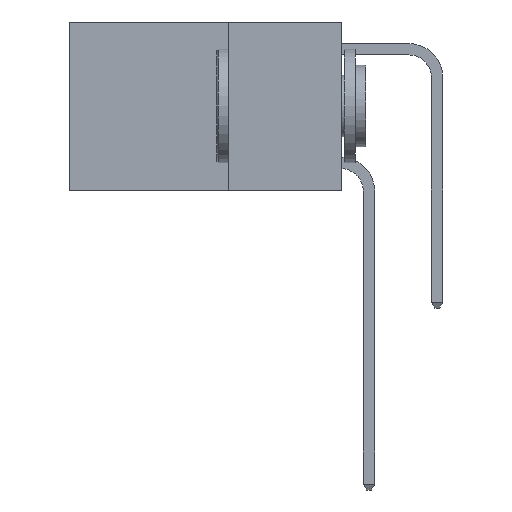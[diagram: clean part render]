
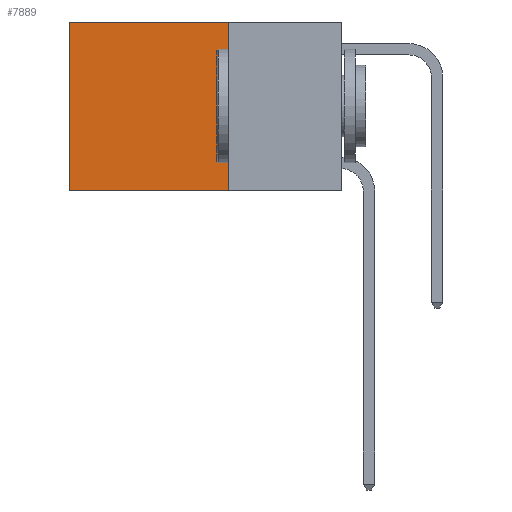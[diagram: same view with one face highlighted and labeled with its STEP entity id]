
A CAD part, left-side view. The second image highlights one B-rep face of the part: STEP entity #7889.
In plain terms, the highlighted planar face has unit normal (-1, 0, 0).
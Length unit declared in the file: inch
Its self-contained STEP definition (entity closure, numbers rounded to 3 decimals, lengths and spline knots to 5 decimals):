
#474 = DIRECTION ( 'NONE',  ( 0., 1., 0. ) ) ;
#716 = AXIS2_PLACEMENT_3D ( 'NONE', #8665, #10063, #4772 ) ;
#807 = PLANE ( 'NONE',  #716 ) ;
#1109 = VERTEX_POINT ( 'NONE', #6477 ) ;
#1209 = EDGE_CURVE ( 'NONE', #4721, #1109, #2411, .T. ) ;
#1441 = ORIENTED_EDGE ( 'NONE', *, *, #4058, .T. ) ;
#1453 = VECTOR ( 'NONE', #474, 39.37008 ) ;
#2411 = LINE ( 'NONE', #10337, #1453 ) ;
#2721 = ORIENTED_EDGE ( 'NONE', *, *, #1209, .F. ) ;
#2748 = EDGE_LOOP ( 'NONE', ( #1441, #2721, #3820, #3314 ) ) ;
#3028 = CARTESIAN_POINT ( 'NONE',  ( 0.2625, 0.25, 0. ) ) ;
#3314 = ORIENTED_EDGE ( 'NONE', *, *, #4713, .T. ) ;
#3820 = ORIENTED_EDGE ( 'NONE', *, *, #5455, .F. ) ;
#3892 = CARTESIAN_POINT ( 'NONE',  ( 0.2625, 0.25, 0. ) ) ;
#4058 = EDGE_CURVE ( 'NONE', #5687, #1109, #5022, .T. ) ;
#4713 = EDGE_CURVE ( 'NONE', #9943, #5687, #7908, .T. ) ;
#4721 = VERTEX_POINT ( 'NONE', #6299 ) ;
#4772 = DIRECTION ( 'NONE',  ( 0., 0., -1. ) ) ;
#4987 = LINE ( 'NONE', #3892, #9052 ) ;
#5022 = LINE ( 'NONE', #8392, #7547 ) ;
#5455 = EDGE_CURVE ( 'NONE', #9943, #4721, #4987, .T. ) ;
#5687 = VERTEX_POINT ( 'NONE', #9915 ) ;
#6299 = CARTESIAN_POINT ( 'NONE',  ( 0.2625, 0.25, -0.37 ) ) ;
#6344 = CARTESIAN_POINT ( 'NONE',  ( 0.2625, 0.25, 0. ) ) ;
#6477 = CARTESIAN_POINT ( 'NONE',  ( 0.2625, 0.6, -0.37 ) ) ;
#7263 = DIRECTION ( 'NONE',  ( 0., 0., -1. ) ) ;
#7494 = FACE_OUTER_BOUND ( 'NONE', #2748, .T. ) ;
#7547 = VECTOR ( 'NONE', #8259, 39.37008 ) ;
#7889 = ADVANCED_FACE ( 'NONE', ( #7494 ), #807, .F. ) ;
#7908 = LINE ( 'NONE', #6344, #9862 ) ;
#8259 = DIRECTION ( 'NONE',  ( 0., 0., -1. ) ) ;
#8392 = CARTESIAN_POINT ( 'NONE',  ( 0.2625, 0.6, 0. ) ) ;
#8665 = CARTESIAN_POINT ( 'NONE',  ( 0.2625, 0.25, 0. ) ) ;
#9052 = VECTOR ( 'NONE', #7263, 39.37008 ) ;
#9862 = VECTOR ( 'NONE', #10190, 39.37008 ) ;
#9915 = CARTESIAN_POINT ( 'NONE',  ( 0.2625, 0.6, 0. ) ) ;
#9943 = VERTEX_POINT ( 'NONE', #3028 ) ;
#10063 = DIRECTION ( 'NONE',  ( 1., 0., 0. ) ) ;
#10190 = DIRECTION ( 'NONE',  ( 0., 1., 0. ) ) ;
#10337 = CARTESIAN_POINT ( 'NONE',  ( 0.2625, 0.25, -0.37 ) ) ;
